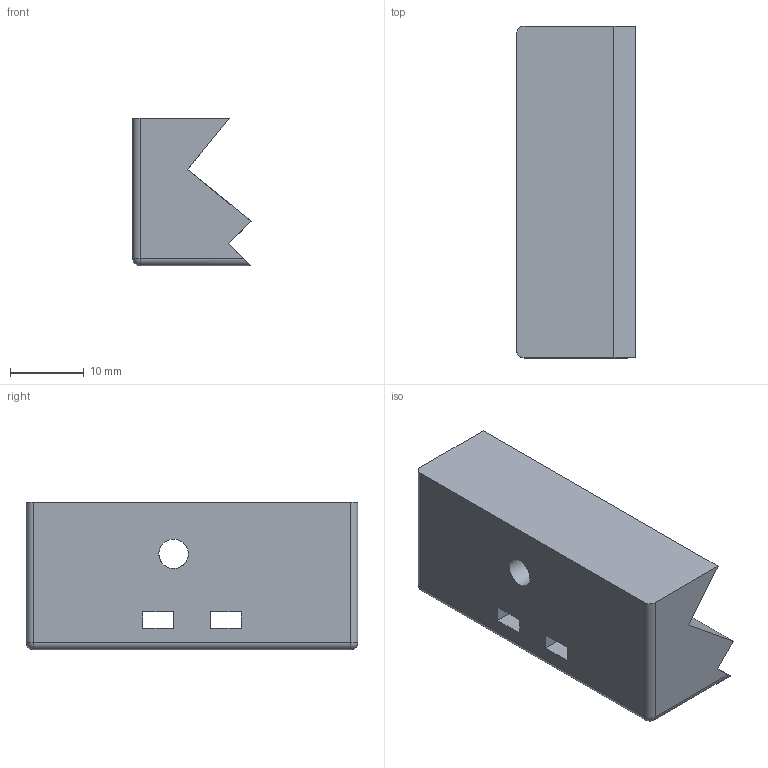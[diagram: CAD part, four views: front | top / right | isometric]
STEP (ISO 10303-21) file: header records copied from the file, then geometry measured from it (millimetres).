
FILE_DESCRIPTION(('FreeCAD Model'),'2;1');
FILE_NAME('V1.1 STL''s & Steps/Left Block V1.1.step','2020-07-30T16:38:21',('Author'),( ''),'Open CASCADE STEP processor 7.3','FreeCAD','Unknown');
FILE_SCHEMA(('AUTOMOTIVE_DESIGN { 1 0 10303 214 1 1 1 1 }'));
Length unit declared in the file: millimetre
Products named in the file (1): BaseFeature001
Bounding box: 16.08 x 45 x 20 mm (x, y, z)
Volume: 10461.5 mm3; surface area: 4324.9 mm2
Topology: 1 solids, 1 shells, 26 faces, 77 edges, 48 vertices
Faces by surface type: plane 18, cylinder 6, sphere 2
Full cylindrical faces by diameter (mm): 4 x1
Entity records: 1899 total; most frequent: CARTESIAN_POINT 368, DIRECTION 284, LINE 198, VECTOR 198, ORIENTED_EDGE 150, PCURVE 150, DEFINITIONAL_REPRESENTATION 150, EDGE_CURVE 75
